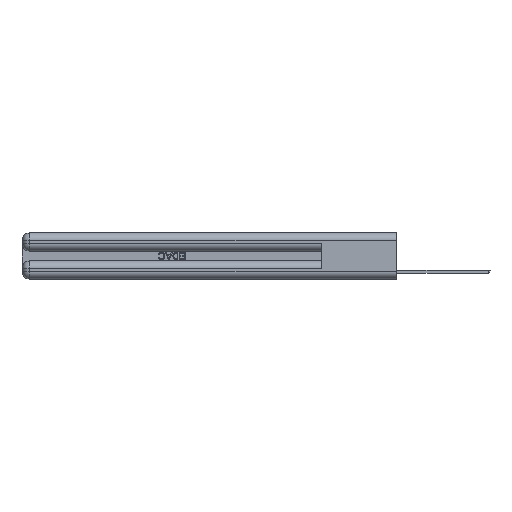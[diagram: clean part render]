
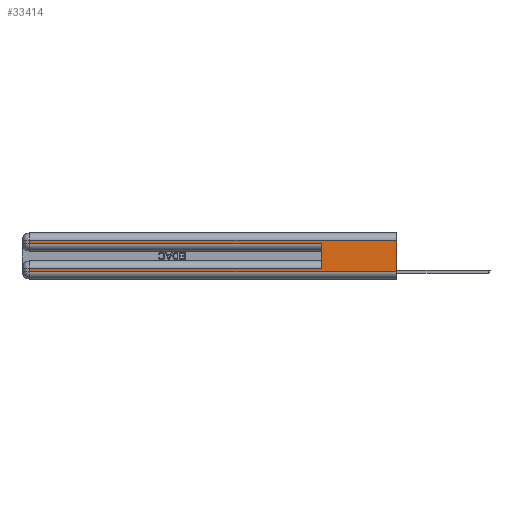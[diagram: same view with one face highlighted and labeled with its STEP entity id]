
A CAD part, left-side view. The second image highlights one B-rep face of the part: STEP entity #33414.
In plain terms, the highlighted planar face has unit normal (-1, 0, 0).
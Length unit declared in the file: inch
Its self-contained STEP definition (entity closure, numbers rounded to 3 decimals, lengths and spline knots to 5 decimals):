
#685 = LINE ( 'NONE', #17255, #20243 ) ;
#696 = VERTEX_POINT ( 'NONE', #6650 ) ;
#1044 = DIRECTION ( 'NONE',  ( 0., 0., -1. ) ) ;
#1050 = ORIENTED_EDGE ( 'NONE', *, *, #4422, .T. ) ;
#1276 = EDGE_CURVE ( 'NONE', #31647, #18236, #35554, .T. ) ;
#1583 = CARTESIAN_POINT ( 'NONE',  ( 0., 0.6, 0.085 ) ) ;
#2091 = VECTOR ( 'NONE', #19217, 39.37008 ) ;
#3864 = CARTESIAN_POINT ( 'NONE',  ( 0., 0., 0.31 ) ) ;
#4422 = EDGE_CURVE ( 'NONE', #14588, #696, #19398, .T. ) ;
#5528 = CARTESIAN_POINT ( 'NONE',  ( 0., 0., 0.06 ) ) ;
#5722 = CARTESIAN_POINT ( 'NONE',  ( 0., 2.94, 0.085 ) ) ;
#6461 = PLANE ( 'NONE',  #33523 ) ;
#6650 = CARTESIAN_POINT ( 'NONE',  ( 0., 0., 0.06 ) ) ;
#7260 = ORIENTED_EDGE ( 'NONE', *, *, #33833, .T. ) ;
#7477 = CARTESIAN_POINT ( 'NONE',  ( 0., 0., 0.285 ) ) ;
#7712 = DIRECTION ( 'NONE',  ( 0., 0., 1. ) ) ;
#7947 = ORIENTED_EDGE ( 'NONE', *, *, #19623, .T. ) ;
#9838 = EDGE_CURVE ( 'NONE', #16545, #16219, #29258, .T. ) ;
#10530 = DIRECTION ( 'NONE',  ( 0., -1., 0. ) ) ;
#10792 = FACE_OUTER_BOUND ( 'NONE', #25920, .T. ) ;
#10922 = DIRECTION ( 'NONE',  ( 0., 1., 0. ) ) ;
#12297 = CARTESIAN_POINT ( 'NONE',  ( 0., 0.6, 0.285 ) ) ;
#12375 = CARTESIAN_POINT ( 'NONE',  ( 0., 2.94, 0.31 ) ) ;
#13331 = VECTOR ( 'NONE', #10530, 39.37008 ) ;
#14205 = DIRECTION ( 'NONE',  ( 1., 0., 0. ) ) ;
#14413 = CARTESIAN_POINT ( 'NONE',  ( 0., 2.94, 0.285 ) ) ;
#14557 = CARTESIAN_POINT ( 'NONE',  ( 0., 0., 0.37 ) ) ;
#14588 = VERTEX_POINT ( 'NONE', #35095 ) ;
#15159 = VECTOR ( 'NONE', #10922, 39.37008 ) ;
#15240 = DIRECTION ( 'NONE',  ( 0., 1., 0. ) ) ;
#16219 = VERTEX_POINT ( 'NONE', #12375 ) ;
#16545 = VERTEX_POINT ( 'NONE', #3864 ) ;
#17255 = CARTESIAN_POINT ( 'NONE',  ( 0., 2.94, 0.37 ) ) ;
#18236 = VERTEX_POINT ( 'NONE', #12297 ) ;
#18875 = CARTESIAN_POINT ( 'NONE',  ( 0., 0.6, 0.145 ) ) ;
#19217 = DIRECTION ( 'NONE',  ( 0., -1., 0. ) ) ;
#19396 = EDGE_CURVE ( 'NONE', #27647, #18236, #30017, .T. ) ;
#19398 = LINE ( 'NONE', #5528, #2091 ) ;
#19623 = EDGE_CURVE ( 'NONE', #23137, #14588, #20815, .T. ) ;
#20243 = VECTOR ( 'NONE', #33451, 39.37008 ) ;
#20378 = ORIENTED_EDGE ( 'NONE', *, *, #9838, .T. ) ;
#20815 = LINE ( 'NONE', #33795, #24685 ) ;
#22815 = DIRECTION ( 'NONE',  ( 0., 0., -1. ) ) ;
#23137 = VERTEX_POINT ( 'NONE', #5722 ) ;
#23915 = DIRECTION ( 'NONE',  ( 0., 0., -1. ) ) ;
#24345 = EDGE_CURVE ( 'NONE', #16545, #696, #29485, .T. ) ;
#24685 = VECTOR ( 'NONE', #22815, 39.37008 ) ;
#24695 = VECTOR ( 'NONE', #15240, 39.37008 ) ;
#25232 = ORIENTED_EDGE ( 'NONE', *, *, #24345, .F. ) ;
#25740 = ORIENTED_EDGE ( 'NONE', *, *, #32112, .T. ) ;
#25920 = EDGE_LOOP ( 'NONE', ( #25232, #20378, #25740, #32481, #29530, #7260, #7947, #1050 ) ) ;
#26762 = LINE ( 'NONE', #29811, #15159 ) ;
#27647 = VERTEX_POINT ( 'NONE', #1583 ) ;
#28870 = VECTOR ( 'NONE', #23915, 39.37008 ) ;
#29258 = LINE ( 'NONE', #35021, #24695 ) ;
#29485 = LINE ( 'NONE', #30204, #28870 ) ;
#29530 = ORIENTED_EDGE ( 'NONE', *, *, #19396, .F. ) ;
#29811 = CARTESIAN_POINT ( 'NONE',  ( 0., 0., 0.085 ) ) ;
#30017 = LINE ( 'NONE', #18875, #33303 ) ;
#30204 = CARTESIAN_POINT ( 'NONE',  ( 0., 0., 0.37 ) ) ;
#31647 = VERTEX_POINT ( 'NONE', #14413 ) ;
#32112 = EDGE_CURVE ( 'NONE', #16219, #31647, #685, .T. ) ;
#32481 = ORIENTED_EDGE ( 'NONE', *, *, #1276, .T. ) ;
#33303 = VECTOR ( 'NONE', #7712, 39.37008 ) ;
#33414 = ADVANCED_FACE ( 'NONE', ( #10792 ), #6461, .F. ) ;
#33451 = DIRECTION ( 'NONE',  ( 0., 0., -1. ) ) ;
#33523 = AXIS2_PLACEMENT_3D ( 'NONE', #14557, #14205, #1044 ) ;
#33795 = CARTESIAN_POINT ( 'NONE',  ( 0., 2.94, 0.37 ) ) ;
#33833 = EDGE_CURVE ( 'NONE', #27647, #23137, #26762, .T. ) ;
#35021 = CARTESIAN_POINT ( 'NONE',  ( 0., 0., 0.31 ) ) ;
#35095 = CARTESIAN_POINT ( 'NONE',  ( 0., 2.94, 0.06 ) ) ;
#35554 = LINE ( 'NONE', #7477, #13331 ) ;
